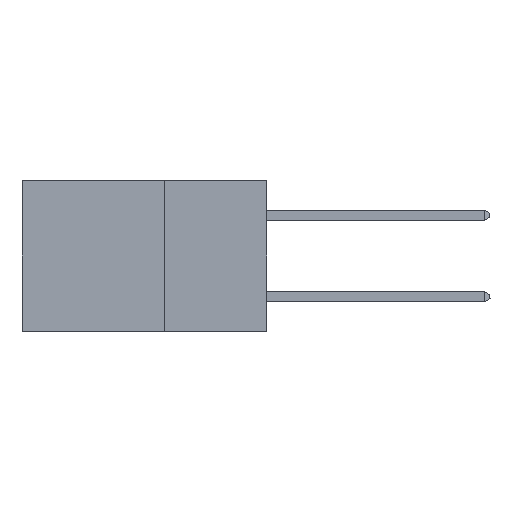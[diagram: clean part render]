
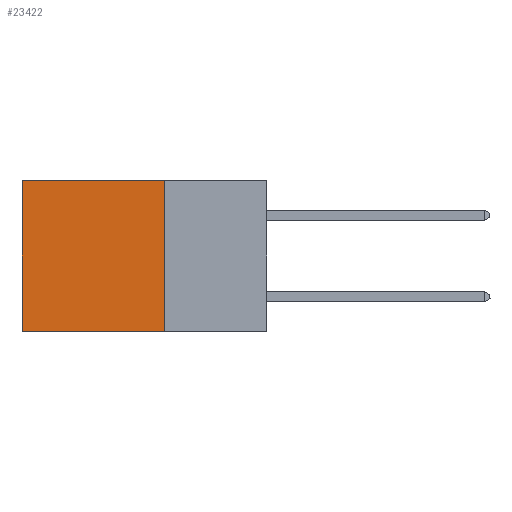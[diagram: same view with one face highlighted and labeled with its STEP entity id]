
A CAD part, left-side view. The second image highlights one B-rep face of the part: STEP entity #23422.
In plain terms, the highlighted planar face has unit normal (-1, 0, 0).
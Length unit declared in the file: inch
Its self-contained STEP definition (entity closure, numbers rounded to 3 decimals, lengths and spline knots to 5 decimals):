
#576 = EDGE_CURVE ( 'NONE', #38970, #22101, #1373, .T. ) ;
#1074 = AXIS2_PLACEMENT_3D ( 'NONE', #33451, #30152, #27507 ) ;
#1373 = LINE ( 'NONE', #24803, #32868 ) ;
#2062 = ORIENTED_EDGE ( 'NONE', *, *, #576, .F. ) ;
#4179 = CARTESIAN_POINT ( 'NONE',  ( 0.2875, 0.25, -0.37 ) ) ;
#6038 = PLANE ( 'NONE',  #1074 ) ;
#7744 = CARTESIAN_POINT ( 'NONE',  ( 0.2875, 0.25, 0. ) ) ;
#8308 = ORIENTED_EDGE ( 'NONE', *, *, #28918, .F. ) ;
#9157 = ORIENTED_EDGE ( 'NONE', *, *, #11656, .T. ) ;
#10045 = VERTEX_POINT ( 'NONE', #7744 ) ;
#11656 = EDGE_CURVE ( 'NONE', #22156, #22101, #21072, .T. ) ;
#12286 = CARTESIAN_POINT ( 'NONE',  ( 0.2875, 0.6, 0. ) ) ;
#17291 = EDGE_CURVE ( 'NONE', #10045, #22156, #36111, .T. ) ;
#21072 = LINE ( 'NONE', #12286, #32081 ) ;
#21181 = CARTESIAN_POINT ( 'NONE',  ( 0.2875, 0.6, -0.37 ) ) ;
#21192 = DIRECTION ( 'NONE',  ( 0., 0., -1. ) ) ;
#22101 = VERTEX_POINT ( 'NONE', #21181 ) ;
#22156 = VERTEX_POINT ( 'NONE', #30419 ) ;
#22830 = ORIENTED_EDGE ( 'NONE', *, *, #17291, .T. ) ;
#23422 = ADVANCED_FACE ( 'NONE', ( #33035 ), #6038, .F. ) ;
#24007 = DIRECTION ( 'NONE',  ( 0., 0., -1. ) ) ;
#24277 = CARTESIAN_POINT ( 'NONE',  ( 0.2875, 0.25, 0. ) ) ;
#24803 = CARTESIAN_POINT ( 'NONE',  ( 0.2875, 0.25, -0.37 ) ) ;
#26649 = VECTOR ( 'NONE', #39274, 39.37008 ) ;
#27507 = DIRECTION ( 'NONE',  ( 0., 0., -1. ) ) ;
#28007 = DIRECTION ( 'NONE',  ( 0., 1., 0. ) ) ;
#28918 = EDGE_CURVE ( 'NONE', #10045, #38970, #32761, .T. ) ;
#29838 = CARTESIAN_POINT ( 'NONE',  ( 0.2875, 0.25, 0. ) ) ;
#30152 = DIRECTION ( 'NONE',  ( 1., 0., 0. ) ) ;
#30419 = CARTESIAN_POINT ( 'NONE',  ( 0.2875, 0.6, 0. ) ) ;
#31187 = EDGE_LOOP ( 'NONE', ( #9157, #2062, #8308, #22830 ) ) ;
#32081 = VECTOR ( 'NONE', #21192, 39.37008 ) ;
#32761 = LINE ( 'NONE', #24277, #36042 ) ;
#32868 = VECTOR ( 'NONE', #28007, 39.37008 ) ;
#33035 = FACE_OUTER_BOUND ( 'NONE', #31187, .T. ) ;
#33451 = CARTESIAN_POINT ( 'NONE',  ( 0.2875, 0.25, 0. ) ) ;
#36042 = VECTOR ( 'NONE', #24007, 39.37008 ) ;
#36111 = LINE ( 'NONE', #29838, #26649 ) ;
#38970 = VERTEX_POINT ( 'NONE', #4179 ) ;
#39274 = DIRECTION ( 'NONE',  ( 0., 1., 0. ) ) ;
